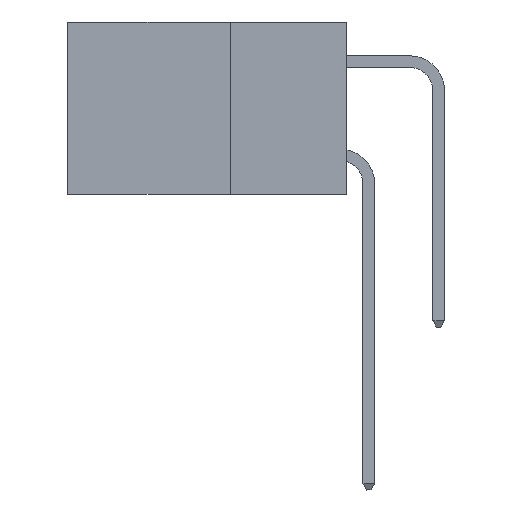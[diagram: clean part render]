
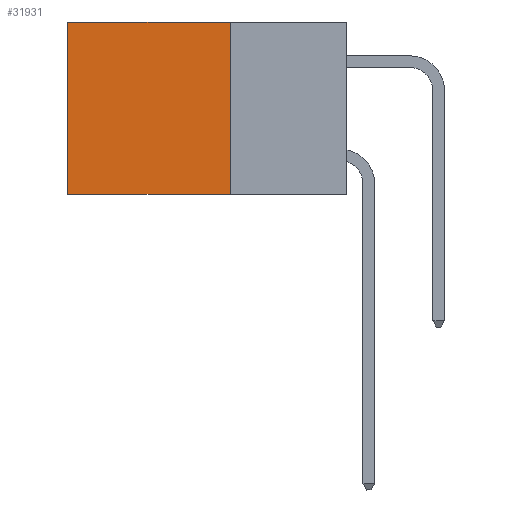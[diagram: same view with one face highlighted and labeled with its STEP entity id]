
A CAD part, left-side view. The second image highlights one B-rep face of the part: STEP entity #31931.
In plain terms, the highlighted planar face has unit normal (-1, 0, 0).
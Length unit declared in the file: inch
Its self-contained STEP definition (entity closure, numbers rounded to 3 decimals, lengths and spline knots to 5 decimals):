
#1087 = CARTESIAN_POINT ( 'NONE',  ( 0.2875, 0.25, 0. ) ) ;
#1345 = CARTESIAN_POINT ( 'NONE',  ( 0.2875, 0.25, -0.37 ) ) ;
#2846 = DIRECTION ( 'NONE',  ( 0., 1., 0. ) ) ;
#3350 = VECTOR ( 'NONE', #20959, 39.37008 ) ;
#3688 = CARTESIAN_POINT ( 'NONE',  ( 0.2875, 0.25, -0.37 ) ) ;
#4153 = LINE ( 'NONE', #29104, #39066 ) ;
#4463 = CARTESIAN_POINT ( 'NONE',  ( 0.2875, 0.6, 0. ) ) ;
#5247 = DIRECTION ( 'NONE',  ( 1., 0., 0. ) ) ;
#5358 = VERTEX_POINT ( 'NONE', #28243 ) ;
#7126 = VECTOR ( 'NONE', #13039, 39.37008 ) ;
#8657 = CARTESIAN_POINT ( 'NONE',  ( 0.2875, 0.6, -0.37 ) ) ;
#8700 = PLANE ( 'NONE',  #34382 ) ;
#11589 = CARTESIAN_POINT ( 'NONE',  ( 0.2875, 0.25, 0. ) ) ;
#11732 = EDGE_CURVE ( 'NONE', #17096, #26135, #14627, .T. ) ;
#12260 = LINE ( 'NONE', #3688, #7126 ) ;
#13039 = DIRECTION ( 'NONE',  ( 0., 1., 0. ) ) ;
#13801 = DIRECTION ( 'NONE',  ( 0., 0., -1. ) ) ;
#14627 = LINE ( 'NONE', #4463, #3350 ) ;
#16861 = LINE ( 'NONE', #1087, #19434 ) ;
#17096 = VERTEX_POINT ( 'NONE', #23866 ) ;
#19434 = VECTOR ( 'NONE', #13801, 39.37008 ) ;
#20947 = EDGE_LOOP ( 'NONE', ( #35430, #29361, #31324, #23812 ) ) ;
#20959 = DIRECTION ( 'NONE',  ( 0., 0., -1. ) ) ;
#23812 = ORIENTED_EDGE ( 'NONE', *, *, #38247, .T. ) ;
#23866 = CARTESIAN_POINT ( 'NONE',  ( 0.2875, 0.6, 0. ) ) ;
#26135 = VERTEX_POINT ( 'NONE', #8657 ) ;
#26520 = EDGE_CURVE ( 'NONE', #5358, #37961, #16861, .T. ) ;
#28243 = CARTESIAN_POINT ( 'NONE',  ( 0.2875, 0.25, 0. ) ) ;
#29104 = CARTESIAN_POINT ( 'NONE',  ( 0.2875, 0.25, 0. ) ) ;
#29361 = ORIENTED_EDGE ( 'NONE', *, *, #32717, .F. ) ;
#31324 = ORIENTED_EDGE ( 'NONE', *, *, #26520, .F. ) ;
#31931 = ADVANCED_FACE ( 'NONE', ( #33410 ), #8700, .F. ) ;
#32717 = EDGE_CURVE ( 'NONE', #37961, #26135, #12260, .T. ) ;
#33410 = FACE_OUTER_BOUND ( 'NONE', #20947, .T. ) ;
#34382 = AXIS2_PLACEMENT_3D ( 'NONE', #11589, #5247, #41534 ) ;
#35430 = ORIENTED_EDGE ( 'NONE', *, *, #11732, .T. ) ;
#37961 = VERTEX_POINT ( 'NONE', #1345 ) ;
#38247 = EDGE_CURVE ( 'NONE', #5358, #17096, #4153, .T. ) ;
#39066 = VECTOR ( 'NONE', #2846, 39.37008 ) ;
#41534 = DIRECTION ( 'NONE',  ( 0., 0., -1. ) ) ;
